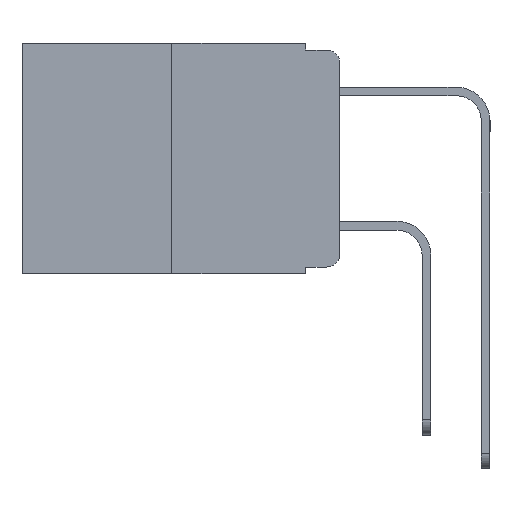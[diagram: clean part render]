
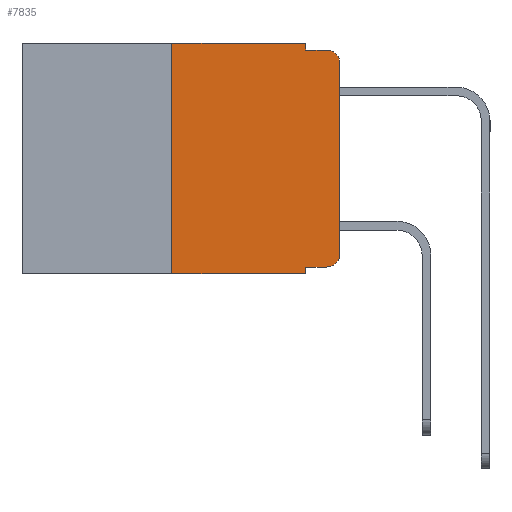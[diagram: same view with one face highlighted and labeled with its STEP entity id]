
A CAD part, left-side view. The second image highlights one B-rep face of the part: STEP entity #7835.
In plain terms, the highlighted planar face has unit normal (-1, 0, 0).
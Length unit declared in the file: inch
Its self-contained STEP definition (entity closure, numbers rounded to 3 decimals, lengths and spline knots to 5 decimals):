
#465 = DIRECTION ( 'NONE',  ( 0., 0., -1. ) ) ;
#491 = LINE ( 'NONE', #6428, #3676 ) ;
#667 = VECTOR ( 'NONE', #12450, 39.37008 ) ;
#826 = VERTEX_POINT ( 'NONE', #4753 ) ;
#1062 = VERTEX_POINT ( 'NONE', #14431 ) ;
#1085 = LINE ( 'NONE', #7217, #12715 ) ;
#1176 = DIRECTION ( 'NONE',  ( -1., 0., 0. ) ) ;
#1178 = DIRECTION ( 'NONE',  ( 0., 0., -1. ) ) ;
#1198 = CARTESIAN_POINT ( 'NONE',  ( 0., 0.473, 0. ) ) ;
#1227 = CARTESIAN_POINT ( 'NONE',  ( 0., 0.051, -0.333 ) ) ;
#1269 = CARTESIAN_POINT ( 'NONE',  ( 0., 0.02, -0.333 ) ) ;
#1994 = VERTEX_POINT ( 'NONE', #1269 ) ;
#2224 = LINE ( 'NONE', #13776, #13054 ) ;
#2335 = DIRECTION ( 'NONE',  ( 0., -1., 0. ) ) ;
#3055 = DIRECTION ( 'NONE',  ( 0., -1., 0. ) ) ;
#3475 = CARTESIAN_POINT ( 'NONE',  ( 0., 0.051, -0.01 ) ) ;
#3676 = VECTOR ( 'NONE', #3055, 39.37008 ) ;
#3817 = LINE ( 'NONE', #1227, #667 ) ;
#4535 = VERTEX_POINT ( 'NONE', #4991 ) ;
#4753 = CARTESIAN_POINT ( 'NONE',  ( 0., 0.051, 0. ) ) ;
#4839 = CARTESIAN_POINT ( 'NONE',  ( 0., 0.473, -0.343 ) ) ;
#4991 = CARTESIAN_POINT ( 'NONE',  ( 0., 0.051, -0.01 ) ) ;
#5256 = LINE ( 'NONE', #3475, #13725 ) ;
#5572 = VERTEX_POINT ( 'NONE', #10043 ) ;
#5631 = LINE ( 'NONE', #9043, #14055 ) ;
#5861 = PLANE ( 'NONE',  #7645 ) ;
#5998 = DIRECTION ( 'NONE',  ( 0., -1., 0. ) ) ;
#6125 = AXIS2_PLACEMENT_3D ( 'NONE', #8009, #1176, #9087 ) ;
#6428 = CARTESIAN_POINT ( 'NONE',  ( 0., 0.473, 0. ) ) ;
#6459 = VERTEX_POINT ( 'NONE', #7921 ) ;
#6854 = LINE ( 'NONE', #8010, #9749 ) ;
#6981 = DIRECTION ( 'NONE',  ( 0., 0., -1. ) ) ;
#7089 = ORIENTED_EDGE ( 'NONE', *, *, #12589, .F. ) ;
#7138 = DIRECTION ( 'NONE',  ( 0., 0., 1. ) ) ;
#7217 = CARTESIAN_POINT ( 'NONE',  ( 0., 0.25, 0. ) ) ;
#7377 = VERTEX_POINT ( 'NONE', #14074 ) ;
#7400 = VECTOR ( 'NONE', #5998, 39.37008 ) ;
#7418 = ORIENTED_EDGE ( 'NONE', *, *, #12544, .T. ) ;
#7442 = DIRECTION ( 'NONE',  ( -1., 0., 0. ) ) ;
#7645 = AXIS2_PLACEMENT_3D ( 'NONE', #1198, #13549, #6981 ) ;
#7731 = LINE ( 'NONE', #4839, #7400 ) ;
#7835 = ADVANCED_FACE ( 'NONE', ( #12940 ), #5861, .F. ) ;
#7921 = CARTESIAN_POINT ( 'NONE',  ( 0., 0.25, 0. ) ) ;
#8009 = CARTESIAN_POINT ( 'NONE',  ( 0., 0.02, -0.03 ) ) ;
#8010 = CARTESIAN_POINT ( 'NONE',  ( 0., 0.051, 0. ) ) ;
#8228 = CIRCLE ( 'NONE', #6125, 0.02 ) ;
#8276 = ORIENTED_EDGE ( 'NONE', *, *, #11795, .F. ) ;
#8444 = ORIENTED_EDGE ( 'NONE', *, *, #12549, .F. ) ;
#8557 = CIRCLE ( 'NONE', #9520, 0.02 ) ;
#9043 = CARTESIAN_POINT ( 'NONE',  ( 0., 0., 0. ) ) ;
#9087 = DIRECTION ( 'NONE',  ( 0., 0., -1. ) ) ;
#9101 = ORIENTED_EDGE ( 'NONE', *, *, #12571, .F. ) ;
#9520 = AXIS2_PLACEMENT_3D ( 'NONE', #13993, #7442, #465 ) ;
#9579 = VERTEX_POINT ( 'NONE', #10882 ) ;
#9749 = VECTOR ( 'NONE', #1178, 39.37008 ) ;
#9941 = ORIENTED_EDGE ( 'NONE', *, *, #12543, .T. ) ;
#10043 = CARTESIAN_POINT ( 'NONE',  ( 0., 0.051, -0.343 ) ) ;
#10417 = DIRECTION ( 'NONE',  ( 0., 0., -1. ) ) ;
#10882 = CARTESIAN_POINT ( 'NONE',  ( 0., 0., -0.03 ) ) ;
#11056 = ORIENTED_EDGE ( 'NONE', *, *, #12612, .T. ) ;
#11288 = DIRECTION ( 'NONE',  ( 0., 0., 1. ) ) ;
#11291 = CARTESIAN_POINT ( 'NONE',  ( 0., 0.02, -0.01 ) ) ;
#11795 = EDGE_CURVE ( 'NONE', #6459, #826, #491, .T. ) ;
#12062 = EDGE_CURVE ( 'NONE', #1062, #5572, #7731, .T. ) ;
#12450 = DIRECTION ( 'NONE',  ( 0., -1., 0. ) ) ;
#12478 = CARTESIAN_POINT ( 'NONE',  ( 0., 0., -0.313 ) ) ;
#12543 = EDGE_CURVE ( 'NONE', #13257, #9579, #5631, .T. ) ;
#12544 = EDGE_CURVE ( 'NONE', #9579, #14401, #8228, .T. ) ;
#12549 = EDGE_CURVE ( 'NONE', #4535, #14401, #5256, .T. ) ;
#12571 = EDGE_CURVE ( 'NONE', #826, #4535, #2224, .T. ) ;
#12589 = EDGE_CURVE ( 'NONE', #1062, #6459, #1085, .T. ) ;
#12593 = EDGE_CURVE ( 'NONE', #7377, #5572, #6854, .T. ) ;
#12612 = EDGE_CURVE ( 'NONE', #7377, #1994, #3817, .T. ) ;
#12715 = VECTOR ( 'NONE', #7138, 39.37008 ) ;
#12876 = EDGE_CURVE ( 'NONE', #1994, #13257, #8557, .T. ) ;
#12940 = FACE_OUTER_BOUND ( 'NONE', #13246, .T. ) ;
#13054 = VECTOR ( 'NONE', #10417, 39.37008 ) ;
#13246 = EDGE_LOOP ( 'NONE', ( #9941, #7418, #8444, #9101, #8276, #7089, #13947, #14248, #11056, #14650 ) ) ;
#13257 = VERTEX_POINT ( 'NONE', #12478 ) ;
#13549 = DIRECTION ( 'NONE',  ( 1., 0., 0. ) ) ;
#13725 = VECTOR ( 'NONE', #2335, 39.37008 ) ;
#13776 = CARTESIAN_POINT ( 'NONE',  ( 0., 0.051, 0. ) ) ;
#13947 = ORIENTED_EDGE ( 'NONE', *, *, #12062, .T. ) ;
#13993 = CARTESIAN_POINT ( 'NONE',  ( 0., 0.02, -0.313 ) ) ;
#14055 = VECTOR ( 'NONE', #11288, 39.37008 ) ;
#14074 = CARTESIAN_POINT ( 'NONE',  ( 0., 0.051, -0.333 ) ) ;
#14248 = ORIENTED_EDGE ( 'NONE', *, *, #12593, .F. ) ;
#14401 = VERTEX_POINT ( 'NONE', #11291 ) ;
#14431 = CARTESIAN_POINT ( 'NONE',  ( 0., 0.25, -0.343 ) ) ;
#14650 = ORIENTED_EDGE ( 'NONE', *, *, #12876, .T. ) ;
